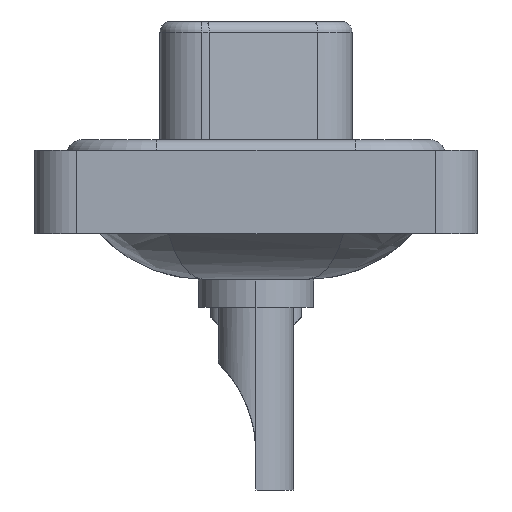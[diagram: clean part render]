
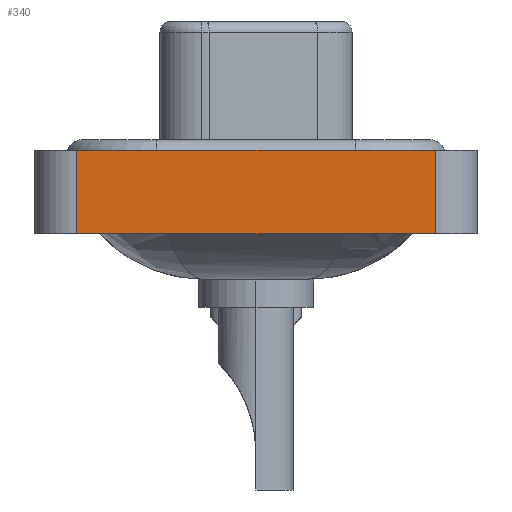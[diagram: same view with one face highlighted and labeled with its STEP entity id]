
A CAD part, left-side view. The second image highlights one B-rep face of the part: STEP entity #340.
In plain terms, the highlighted planar face has unit normal (-1, 0, 0).
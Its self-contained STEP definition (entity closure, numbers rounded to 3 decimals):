
#340 = ADVANCED_FACE ( 'NONE', ( #1528 ), #8470, .T. ) ;
#785 = DIRECTION ( 'NONE',  ( 0., -1., 0. ) ) ;
#1356 = VECTOR ( 'NONE', #9307, 1000. ) ;
#1528 = FACE_OUTER_BOUND ( 'NONE', #19840, .T. ) ;
#2439 = CARTESIAN_POINT ( 'NONE',  ( -7.35, 8.55, -3.6 ) ) ;
#2488 = LINE ( 'NONE', #5639, #1356 ) ;
#2510 = ORIENTED_EDGE ( 'NONE', *, *, #8138, .F. ) ;
#2747 = VERTEX_POINT ( 'NONE', #2439 ) ;
#2816 = DIRECTION ( 'NONE',  ( 0., 0., 1. ) ) ;
#3612 = CARTESIAN_POINT ( 'NONE',  ( -7.35, -8.55, 0.4 ) ) ;
#4378 = EDGE_CURVE ( 'NONE', #2747, #8649, #19537, .T. ) ;
#5639 = CARTESIAN_POINT ( 'NONE',  ( -7.35, -8.55, -3.6 ) ) ;
#5697 = CARTESIAN_POINT ( 'NONE',  ( -7.35, -8.55, 0.4 ) ) ;
#6629 = DIRECTION ( 'NONE',  ( 0., 0., 1. ) ) ;
#7415 = VERTEX_POINT ( 'NONE', #15173 ) ;
#8138 = EDGE_CURVE ( 'NONE', #8649, #10817, #10460, .T. ) ;
#8470 = PLANE ( 'NONE',  #16122 ) ;
#8649 = VERTEX_POINT ( 'NONE', #12146 ) ;
#9010 = LINE ( 'NONE', #15583, #20086 ) ;
#9307 = DIRECTION ( 'NONE',  ( 0., 0., 1. ) ) ;
#9445 = ORIENTED_EDGE ( 'NONE', *, *, #17823, .T. ) ;
#9881 = VECTOR ( 'NONE', #17036, 1000. ) ;
#10460 = LINE ( 'NONE', #5697, #9881 ) ;
#10817 = VERTEX_POINT ( 'NONE', #3612 ) ;
#11477 = CARTESIAN_POINT ( 'NONE',  ( -7.35, -8.55, -3.6 ) ) ;
#12146 = CARTESIAN_POINT ( 'NONE',  ( -7.35, 8.55, 0.4 ) ) ;
#13073 = DIRECTION ( 'NONE',  ( -1., 0., 0. ) ) ;
#13415 = ORIENTED_EDGE ( 'NONE', *, *, #4378, .F. ) ;
#14926 = ORIENTED_EDGE ( 'NONE', *, *, #19599, .T. ) ;
#15173 = CARTESIAN_POINT ( 'NONE',  ( -7.35, -8.55, -3.6 ) ) ;
#15583 = CARTESIAN_POINT ( 'NONE',  ( -7.35, -8.55, -3.6 ) ) ;
#15988 = CARTESIAN_POINT ( 'NONE',  ( -7.35, 8.55, -3.6 ) ) ;
#16122 = AXIS2_PLACEMENT_3D ( 'NONE', #11477, #13073, #6629 ) ;
#16591 = VECTOR ( 'NONE', #2816, 1000. ) ;
#17036 = DIRECTION ( 'NONE',  ( 0., -1., 0. ) ) ;
#17823 = EDGE_CURVE ( 'NONE', #2747, #7415, #9010, .T. ) ;
#19537 = LINE ( 'NONE', #15988, #16591 ) ;
#19599 = EDGE_CURVE ( 'NONE', #7415, #10817, #2488, .T. ) ;
#19840 = EDGE_LOOP ( 'NONE', ( #14926, #2510, #13415, #9445 ) ) ;
#20086 = VECTOR ( 'NONE', #785, 1000. ) ;
